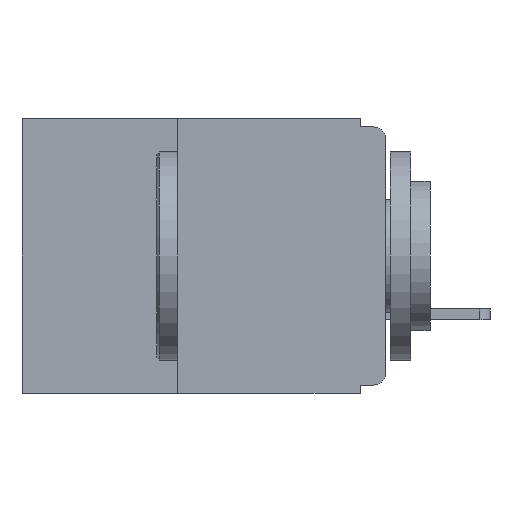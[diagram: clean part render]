
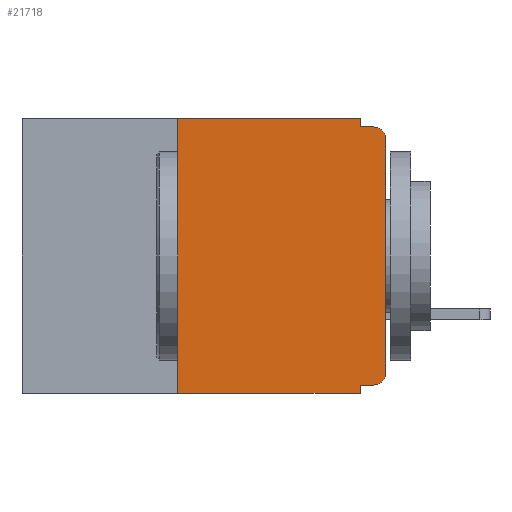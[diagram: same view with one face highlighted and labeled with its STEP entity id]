
A CAD part, left-side view. The second image highlights one B-rep face of the part: STEP entity #21718.
In plain terms, the highlighted planar face has unit normal (-1, 0, 0).
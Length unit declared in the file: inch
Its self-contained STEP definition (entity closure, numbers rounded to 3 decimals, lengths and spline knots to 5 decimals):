
#508 = VECTOR ( 'NONE', #4934, 39.37008 ) ;
#1130 = DIRECTION ( 'NONE',  ( 0., 0., -1. ) ) ;
#1498 = VERTEX_POINT ( 'NONE', #15570 ) ;
#2208 = LINE ( 'NONE', #4607, #17928 ) ;
#2564 = LINE ( 'NONE', #26388, #8363 ) ;
#3164 = CARTESIAN_POINT ( 'NONE',  ( 0., 0.25, -0.33 ) ) ;
#3173 = VECTOR ( 'NONE', #12984, 39.37008 ) ;
#3174 = EDGE_CURVE ( 'NONE', #20158, #4046, #23877, .T. ) ;
#3314 = LINE ( 'NONE', #7230, #14092 ) ;
#3696 = EDGE_CURVE ( 'NONE', #11347, #23055, #12079, .T. ) ;
#4046 = VERTEX_POINT ( 'NONE', #23662 ) ;
#4441 = VERTEX_POINT ( 'NONE', #15840 ) ;
#4514 = VECTOR ( 'NONE', #25736, 39.37008 ) ;
#4607 = CARTESIAN_POINT ( 'NONE',  ( 0., 0.031, 0. ) ) ;
#4934 = DIRECTION ( 'NONE',  ( 0., -1., 0. ) ) ;
#5139 = DIRECTION ( 'NONE',  ( 0., 0., 1. ) ) ;
#5371 = ORIENTED_EDGE ( 'NONE', *, *, #14859, .F. ) ;
#6190 = EDGE_CURVE ( 'NONE', #12343, #4046, #11594, .T. ) ;
#6757 = ORIENTED_EDGE ( 'NONE', *, *, #19433, .F. ) ;
#6760 = DIRECTION ( 'NONE',  ( 1., 0., 0. ) ) ;
#7230 = CARTESIAN_POINT ( 'NONE',  ( 0., 0.437, 0. ) ) ;
#7298 = CARTESIAN_POINT ( 'NONE',  ( 0., 0., -0.025 ) ) ;
#8054 = ORIENTED_EDGE ( 'NONE', *, *, #3696, .T. ) ;
#8363 = VECTOR ( 'NONE', #11778, 39.37008 ) ;
#8457 = CARTESIAN_POINT ( 'NONE',  ( 0., 0.437, 0. ) ) ;
#8519 = VERTEX_POINT ( 'NONE', #16422 ) ;
#8923 = EDGE_CURVE ( 'NONE', #11347, #8519, #23790, .T. ) ;
#9122 = CARTESIAN_POINT ( 'NONE',  ( 0., 0., -0.305 ) ) ;
#9580 = CIRCLE ( 'NONE', #22059, 0.015 ) ;
#10172 = CARTESIAN_POINT ( 'NONE',  ( 0., 0.031, 0. ) ) ;
#10940 = FACE_OUTER_BOUND ( 'NONE', #15651, .T. ) ;
#11347 = VERTEX_POINT ( 'NONE', #3164 ) ;
#11489 = VERTEX_POINT ( 'NONE', #10172 ) ;
#11594 = LINE ( 'NONE', #25771, #4514 ) ;
#11778 = DIRECTION ( 'NONE',  ( 0., 0., 1. ) ) ;
#11964 = ORIENTED_EDGE ( 'NONE', *, *, #25434, .T. ) ;
#11976 = ORIENTED_EDGE ( 'NONE', *, *, #16732, .F. ) ;
#12079 = LINE ( 'NONE', #22766, #508 ) ;
#12343 = VERTEX_POINT ( 'NONE', #13288 ) ;
#12664 = VECTOR ( 'NONE', #5139, 39.37008 ) ;
#12984 = DIRECTION ( 'NONE',  ( 0., 0., -1. ) ) ;
#13288 = CARTESIAN_POINT ( 'NONE',  ( 0., 0.031, -0.01 ) ) ;
#14071 = DIRECTION ( 'NONE',  ( -1., 0., 0. ) ) ;
#14092 = VECTOR ( 'NONE', #17791, 39.37008 ) ;
#14669 = CARTESIAN_POINT ( 'NONE',  ( 0., 0., -0.32 ) ) ;
#14756 = DIRECTION ( 'NONE',  ( 0., 1., 0. ) ) ;
#14827 = LINE ( 'NONE', #14669, #19690 ) ;
#14859 = EDGE_CURVE ( 'NONE', #1498, #23055, #24376, .T. ) ;
#14876 = PLANE ( 'NONE',  #20416 ) ;
#15275 = ORIENTED_EDGE ( 'NONE', *, *, #17645, .F. ) ;
#15570 = CARTESIAN_POINT ( 'NONE',  ( 0., 0.031, -0.32 ) ) ;
#15651 = EDGE_LOOP ( 'NONE', ( #11964, #16073, #16243, #6757, #15275, #18353, #8054, #5371, #11976, #24667 ) ) ;
#15665 = EDGE_CURVE ( 'NONE', #4441, #16057, #9580, .T. ) ;
#15840 = CARTESIAN_POINT ( 'NONE',  ( 0., 0.015, -0.32 ) ) ;
#16057 = VERTEX_POINT ( 'NONE', #9122 ) ;
#16073 = ORIENTED_EDGE ( 'NONE', *, *, #3174, .T. ) ;
#16243 = ORIENTED_EDGE ( 'NONE', *, *, #6190, .F. ) ;
#16422 = CARTESIAN_POINT ( 'NONE',  ( 0., 0.25, 0. ) ) ;
#16732 = EDGE_CURVE ( 'NONE', #4441, #1498, #14827, .T. ) ;
#17645 = EDGE_CURVE ( 'NONE', #8519, #11489, #3314, .T. ) ;
#17791 = DIRECTION ( 'NONE',  ( 0., -1., 0. ) ) ;
#17857 = CARTESIAN_POINT ( 'NONE',  ( 0., 0.25, -0.33 ) ) ;
#17928 = VECTOR ( 'NONE', #19528, 39.37008 ) ;
#18353 = ORIENTED_EDGE ( 'NONE', *, *, #8923, .F. ) ;
#19433 = EDGE_CURVE ( 'NONE', #11489, #12343, #2208, .T. ) ;
#19528 = DIRECTION ( 'NONE',  ( 0., 0., -1. ) ) ;
#19690 = VECTOR ( 'NONE', #14756, 39.37008 ) ;
#20158 = VERTEX_POINT ( 'NONE', #7298 ) ;
#20416 = AXIS2_PLACEMENT_3D ( 'NONE', #8457, #6760, #21521 ) ;
#21521 = DIRECTION ( 'NONE',  ( 0., 0., -1. ) ) ;
#21604 = AXIS2_PLACEMENT_3D ( 'NONE', #23935, #23958, #23813 ) ;
#21718 = ADVANCED_FACE ( 'NONE', ( #10940 ), #14876, .F. ) ;
#22059 = AXIS2_PLACEMENT_3D ( 'NONE', #26548, #14071, #1130 ) ;
#22766 = CARTESIAN_POINT ( 'NONE',  ( 0., 0.437, -0.33 ) ) ;
#23055 = VERTEX_POINT ( 'NONE', #24155 ) ;
#23662 = CARTESIAN_POINT ( 'NONE',  ( 0., 0.015, -0.01 ) ) ;
#23790 = LINE ( 'NONE', #17857, #12664 ) ;
#23813 = DIRECTION ( 'NONE',  ( 0., 0., -1. ) ) ;
#23877 = CIRCLE ( 'NONE', #21604, 0.015 ) ;
#23935 = CARTESIAN_POINT ( 'NONE',  ( 0., 0.015, -0.025 ) ) ;
#23958 = DIRECTION ( 'NONE',  ( -1., 0., 0. ) ) ;
#24155 = CARTESIAN_POINT ( 'NONE',  ( 0., 0.031, -0.33 ) ) ;
#24376 = LINE ( 'NONE', #25489, #3173 ) ;
#24667 = ORIENTED_EDGE ( 'NONE', *, *, #15665, .T. ) ;
#25434 = EDGE_CURVE ( 'NONE', #16057, #20158, #2564, .T. ) ;
#25489 = CARTESIAN_POINT ( 'NONE',  ( 0., 0.031, -0.33 ) ) ;
#25736 = DIRECTION ( 'NONE',  ( 0., -1., 0. ) ) ;
#25771 = CARTESIAN_POINT ( 'NONE',  ( 0., 0., -0.01 ) ) ;
#26388 = CARTESIAN_POINT ( 'NONE',  ( 0., 0., 0. ) ) ;
#26548 = CARTESIAN_POINT ( 'NONE',  ( 0., 0.015, -0.305 ) ) ;
